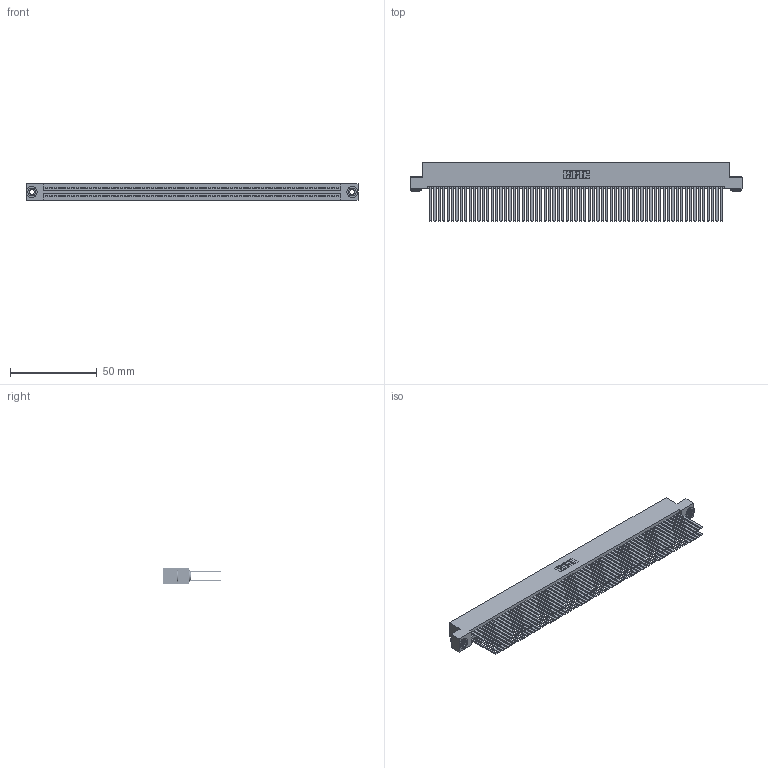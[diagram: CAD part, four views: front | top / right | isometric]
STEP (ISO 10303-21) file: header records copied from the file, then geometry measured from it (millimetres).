
FILE_DESCRIPTION (( 'STEP AP203' ), '1' );
FILE_NAME ('345-134-544-203.STEP', '2019-11-08T03:08:54', ( '' ), ( '' ), 'SwSTEP 2.0', 'SolidWorks 2016', '' );
FILE_SCHEMA (( 'CONFIG_CONTROL_DESIGN' ));
Length unit declared in the file: inch
Products named in the file (4): 345 Part_Flush Mounting Lugs - 0.156 Dia-TH; 345-250-002_345-250-002-102; 345-134-544-203; 345-292-001_345-293-144
Assembly tree (137 placements, depth 2):
  345-134-544-203
    345 Part_Flush Mounting Lugs - 0.156 Dia-TH
    345-292-001_345-293-144  x134
    345-250-002_345-250-002-102  x2
Bounding box: 191.39 x 33.96 x 9.4 mm (x, y, z)
Volume: 20721.6 mm3; surface area: 36824.6 mm2
Topology: 137 solids, 137 shells, 6060 faces, 17971 edges, 11798 vertices
Faces by surface type: plane 3976, cylinder 2076, cone 8
Entity records: 49670 total; most frequent: CARTESIAN_POINT 8275, ORIENTED_EDGE 8202, DIRECTION 7295, EDGE_CURVE 4101, LINE 3681, VECTOR 3681, VERTEX_POINT 2730, AXIS2_PLACEMENT_3D 1807
